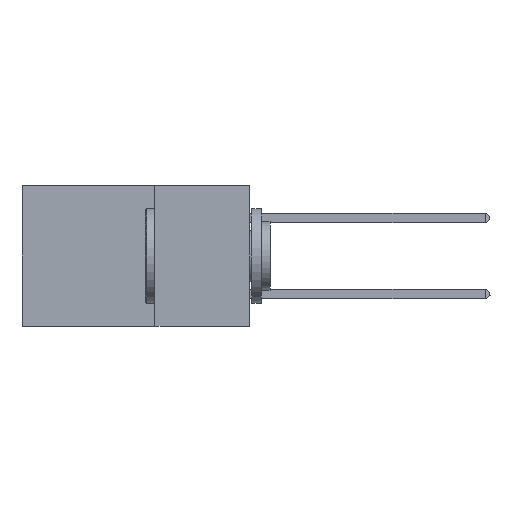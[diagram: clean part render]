
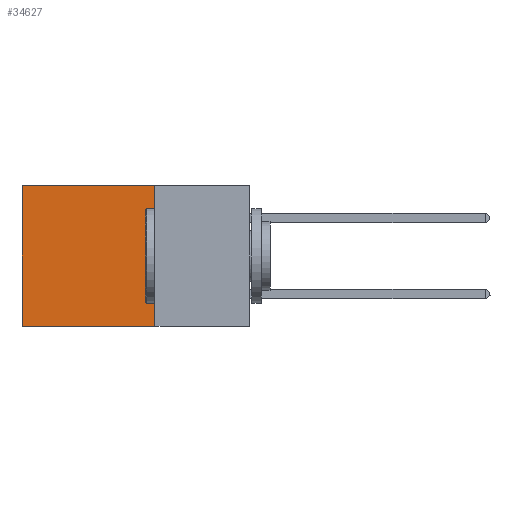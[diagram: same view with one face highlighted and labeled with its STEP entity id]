
A CAD part, left-side view. The second image highlights one B-rep face of the part: STEP entity #34627.
In plain terms, the highlighted planar face has unit normal (-1, 0, 0).
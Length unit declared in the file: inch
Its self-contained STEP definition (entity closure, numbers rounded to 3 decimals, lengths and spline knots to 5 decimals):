
#2878 = EDGE_CURVE ( 'NONE', #40564, #10850, #23106, .T. ) ;
#3624 = CARTESIAN_POINT ( 'NONE',  ( 0.2875, 0.6, 0. ) ) ;
#4085 = ORIENTED_EDGE ( 'NONE', *, *, #21031, .F. ) ;
#5094 = LINE ( 'NONE', #24620, #29261 ) ;
#5976 = CARTESIAN_POINT ( 'NONE',  ( 0.2875, 0.25, 0. ) ) ;
#6320 = LINE ( 'NONE', #31898, #39149 ) ;
#6697 = EDGE_CURVE ( 'NONE', #10850, #19542, #16307, .T. ) ;
#7459 = DIRECTION ( 'NONE',  ( 0., 1., 0. ) ) ;
#8494 = VECTOR ( 'NONE', #20255, 39.37008 ) ;
#9337 = DIRECTION ( 'NONE',  ( 0., 0., -1. ) ) ;
#10850 = VERTEX_POINT ( 'NONE', #3624 ) ;
#11742 = DIRECTION ( 'NONE',  ( 0., 0., -1. ) ) ;
#16307 = LINE ( 'NONE', #16978, #8494 ) ;
#16978 = CARTESIAN_POINT ( 'NONE',  ( 0.2875, 0.6, 0. ) ) ;
#18969 = DIRECTION ( 'NONE',  ( 0., 1., 0. ) ) ;
#19105 = ORIENTED_EDGE ( 'NONE', *, *, #2878, .T. ) ;
#19542 = VERTEX_POINT ( 'NONE', #27420 ) ;
#20255 = DIRECTION ( 'NONE',  ( 0., 0., -1. ) ) ;
#21031 = EDGE_CURVE ( 'NONE', #40564, #24744, #5094, .T. ) ;
#23106 = LINE ( 'NONE', #30399, #31736 ) ;
#24620 = CARTESIAN_POINT ( 'NONE',  ( 0.2875, 0.25, 0. ) ) ;
#24744 = VERTEX_POINT ( 'NONE', #29029 ) ;
#26980 = EDGE_CURVE ( 'NONE', #24744, #19542, #6320, .T. ) ;
#27420 = CARTESIAN_POINT ( 'NONE',  ( 0.2875, 0.6, -0.37 ) ) ;
#28939 = DIRECTION ( 'NONE',  ( 1., 0., 0. ) ) ;
#29029 = CARTESIAN_POINT ( 'NONE',  ( 0.2875, 0.25, -0.37 ) ) ;
#29261 = VECTOR ( 'NONE', #11742, 39.37008 ) ;
#29690 = EDGE_LOOP ( 'NONE', ( #38182, #31298, #4085, #19105 ) ) ;
#30399 = CARTESIAN_POINT ( 'NONE',  ( 0.2875, 0.25, 0. ) ) ;
#31298 = ORIENTED_EDGE ( 'NONE', *, *, #26980, .F. ) ;
#31736 = VECTOR ( 'NONE', #7459, 39.37008 ) ;
#31898 = CARTESIAN_POINT ( 'NONE',  ( 0.2875, 0.25, -0.37 ) ) ;
#32085 = PLANE ( 'NONE',  #42125 ) ;
#34627 = ADVANCED_FACE ( 'NONE', ( #42633 ), #32085, .F. ) ;
#35111 = CARTESIAN_POINT ( 'NONE',  ( 0.2875, 0.25, 0. ) ) ;
#38182 = ORIENTED_EDGE ( 'NONE', *, *, #6697, .T. ) ;
#39149 = VECTOR ( 'NONE', #18969, 39.37008 ) ;
#40564 = VERTEX_POINT ( 'NONE', #35111 ) ;
#42125 = AXIS2_PLACEMENT_3D ( 'NONE', #5976, #28939, #9337 ) ;
#42633 = FACE_OUTER_BOUND ( 'NONE', #29690, .T. ) ;
